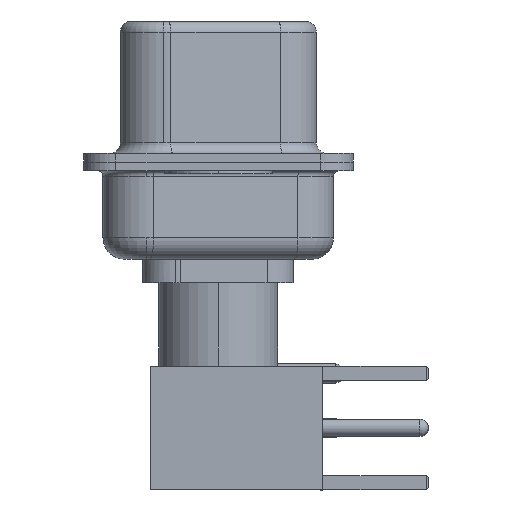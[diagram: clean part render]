
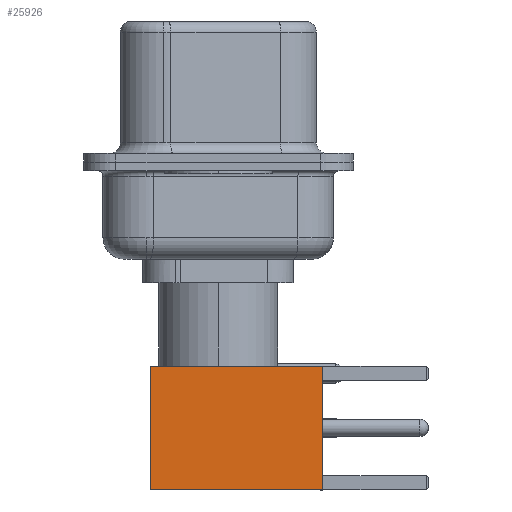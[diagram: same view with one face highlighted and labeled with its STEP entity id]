
A CAD part, left-side view. The second image highlights one B-rep face of the part: STEP entity #25926.
In plain terms, the highlighted face is planar.
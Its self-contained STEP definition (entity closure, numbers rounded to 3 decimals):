
#276 = LINE ( 'NONE', #2346, #20648 ) ;
#1887 = VERTEX_POINT ( 'NONE', #6684 ) ;
#2346 = CARTESIAN_POINT ( 'NONE',  ( -2.875, 2.875, 0. ) ) ;
#6684 = CARTESIAN_POINT ( 'NONE',  ( -2.875, 2.875, 0. ) ) ;
#8971 = DIRECTION ( 'NONE',  ( 0., 0., -1. ) ) ;
#9233 = VERTEX_POINT ( 'NONE', #19758 ) ;
#9743 = CARTESIAN_POINT ( 'NONE',  ( 0., 2.875, 0. ) ) ;
#10880 = FACE_OUTER_BOUND ( 'NONE', #21833, .T. ) ;
#11026 = CARTESIAN_POINT ( 'NONE',  ( 2.875, 2.875, 0. ) ) ;
#11717 = VECTOR ( 'NONE', #20147, 1000. ) ;
#11889 = ORIENTED_EDGE ( 'NONE', *, *, #25893, .T. ) ;
#12734 = EDGE_CURVE ( 'NONE', #16274, #28507, #16327, .T. ) ;
#13047 = EDGE_CURVE ( 'NONE', #16274, #9233, #13508, .T. ) ;
#13065 = EDGE_CURVE ( 'NONE', #28507, #1887, #276, .T. ) ;
#13508 = LINE ( 'NONE', #18067, #11717 ) ;
#15439 = PLANE ( 'NONE',  #16999 ) ;
#16274 = VERTEX_POINT ( 'NONE', #27886 ) ;
#16327 = LINE ( 'NONE', #25305, #17008 ) ;
#16956 = CARTESIAN_POINT ( 'NONE',  ( -2.875, 2.875, 8. ) ) ;
#16999 = AXIS2_PLACEMENT_3D ( 'NONE', #11026, #26474, #20152 ) ;
#17008 = VECTOR ( 'NONE', #25747, 1000. ) ;
#18067 = CARTESIAN_POINT ( 'NONE',  ( 2.875, 2.875, 0. ) ) ;
#18721 = DIRECTION ( 'NONE',  ( -1., 0., 0. ) ) ;
#19758 = CARTESIAN_POINT ( 'NONE',  ( 2.875, 2.875, 0. ) ) ;
#19828 = VECTOR ( 'NONE', #18721, 1000. ) ;
#20147 = DIRECTION ( 'NONE',  ( 0., 0., -1. ) ) ;
#20152 = DIRECTION ( 'NONE',  ( 0., 0., 1. ) ) ;
#20338 = ORIENTED_EDGE ( 'NONE', *, *, #13047, .T. ) ;
#20648 = VECTOR ( 'NONE', #8971, 1000. ) ;
#21833 = EDGE_LOOP ( 'NONE', ( #20338, #11889, #25059, #27747 ) ) ;
#23133 = LINE ( 'NONE', #9743, #19828 ) ;
#25059 = ORIENTED_EDGE ( 'NONE', *, *, #13065, .F. ) ;
#25305 = CARTESIAN_POINT ( 'NONE',  ( 0., 2.875, 8. ) ) ;
#25747 = DIRECTION ( 'NONE',  ( -1., 0., 0. ) ) ;
#25893 = EDGE_CURVE ( 'NONE', #9233, #1887, #23133, .T. ) ;
#25926 = ADVANCED_FACE ( 'NONE', ( #10880 ), #15439, .T. ) ;
#26474 = DIRECTION ( 'NONE',  ( 0., 1., 0. ) ) ;
#27747 = ORIENTED_EDGE ( 'NONE', *, *, #12734, .F. ) ;
#27886 = CARTESIAN_POINT ( 'NONE',  ( 2.875, 2.875, 8. ) ) ;
#28507 = VERTEX_POINT ( 'NONE', #16956 ) ;
